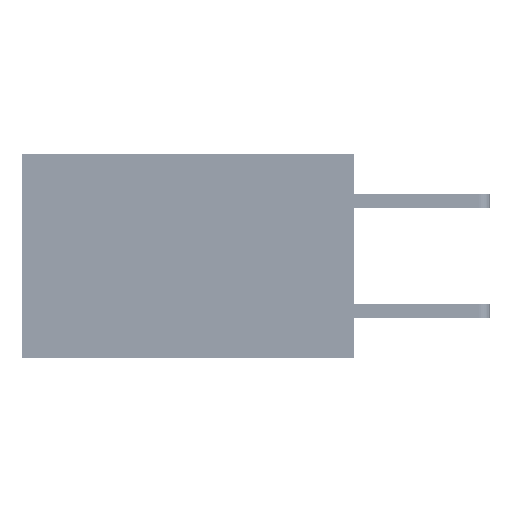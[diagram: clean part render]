
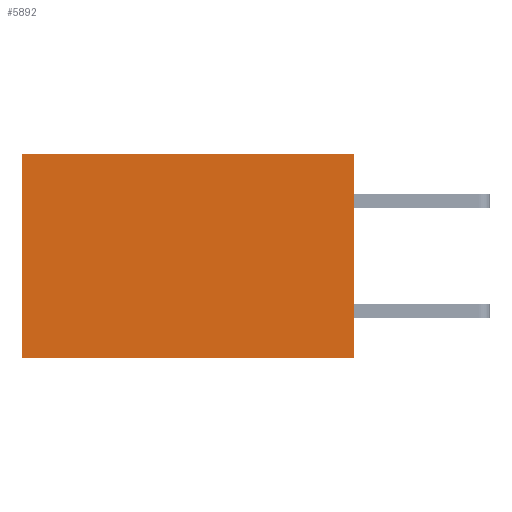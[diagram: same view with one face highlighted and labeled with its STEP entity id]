
A CAD part, left-side view. The second image highlights one B-rep face of the part: STEP entity #5892.
In plain terms, the highlighted planar face has unit normal (-1, 0, 0).
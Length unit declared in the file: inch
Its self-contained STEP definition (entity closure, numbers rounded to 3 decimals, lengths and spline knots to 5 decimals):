
#385 = DIRECTION ( 'NONE',  ( 1., 0., 0. ) ) ;
#1319 = LINE ( 'NONE', #8776, #31363 ) ;
#2233 = EDGE_LOOP ( 'NONE', ( #16275, #9616, #7023, #11544 ) ) ;
#2347 = CARTESIAN_POINT ( 'NONE',  ( 0.2875, 0., 0. ) ) ;
#3647 = LINE ( 'NONE', #15268, #23700 ) ;
#3751 = DIRECTION ( 'NONE',  ( 0., 0., -1. ) ) ;
#5127 = CARTESIAN_POINT ( 'NONE',  ( 0.2875, 0., 0. ) ) ;
#5892 = ADVANCED_FACE ( 'NONE', ( #43095 ), #7126, .F. ) ;
#6822 = CARTESIAN_POINT ( 'NONE',  ( 0.2875, 0., 0. ) ) ;
#7023 = ORIENTED_EDGE ( 'NONE', *, *, #34075, .F. ) ;
#7126 = PLANE ( 'NONE',  #24575 ) ;
#8776 = CARTESIAN_POINT ( 'NONE',  ( 0.2875, 0., -0.37 ) ) ;
#9418 = EDGE_CURVE ( 'NONE', #40077, #42674, #21006, .T. ) ;
#9616 = ORIENTED_EDGE ( 'NONE', *, *, #32772, .F. ) ;
#11240 = LINE ( 'NONE', #29032, #31281 ) ;
#11544 = ORIENTED_EDGE ( 'NONE', *, *, #9418, .T. ) ;
#15268 = CARTESIAN_POINT ( 'NONE',  ( 0.2875, 0.6, 0. ) ) ;
#16275 = ORIENTED_EDGE ( 'NONE', *, *, #37915, .T. ) ;
#17992 = VERTEX_POINT ( 'NONE', #42491 ) ;
#20617 = VERTEX_POINT ( 'NONE', #27440 ) ;
#21006 = LINE ( 'NONE', #5127, #36842 ) ;
#23700 = VECTOR ( 'NONE', #38931, 39.37008 ) ;
#24575 = AXIS2_PLACEMENT_3D ( 'NONE', #6822, #385, #3751 ) ;
#27440 = CARTESIAN_POINT ( 'NONE',  ( 0.2875, 0., -0.37 ) ) ;
#29032 = CARTESIAN_POINT ( 'NONE',  ( 0.2875, 0., 0. ) ) ;
#29579 = DIRECTION ( 'NONE',  ( 0., 1., 0. ) ) ;
#31281 = VECTOR ( 'NONE', #32563, 39.37008 ) ;
#31363 = VECTOR ( 'NONE', #29579, 39.37008 ) ;
#32486 = CARTESIAN_POINT ( 'NONE',  ( 0.2875, 0.6, 0. ) ) ;
#32563 = DIRECTION ( 'NONE',  ( 0., 0., -1. ) ) ;
#32772 = EDGE_CURVE ( 'NONE', #20617, #17992, #1319, .T. ) ;
#34075 = EDGE_CURVE ( 'NONE', #40077, #20617, #11240, .T. ) ;
#35518 = DIRECTION ( 'NONE',  ( 0., 1., 0. ) ) ;
#36842 = VECTOR ( 'NONE', #35518, 39.37008 ) ;
#37915 = EDGE_CURVE ( 'NONE', #42674, #17992, #3647, .T. ) ;
#38931 = DIRECTION ( 'NONE',  ( 0., 0., -1. ) ) ;
#40077 = VERTEX_POINT ( 'NONE', #2347 ) ;
#42491 = CARTESIAN_POINT ( 'NONE',  ( 0.2875, 0.6, -0.37 ) ) ;
#42674 = VERTEX_POINT ( 'NONE', #32486 ) ;
#43095 = FACE_OUTER_BOUND ( 'NONE', #2233, .T. ) ;
